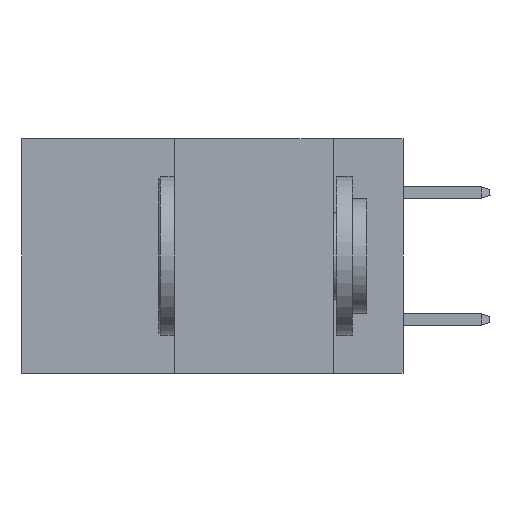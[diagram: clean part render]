
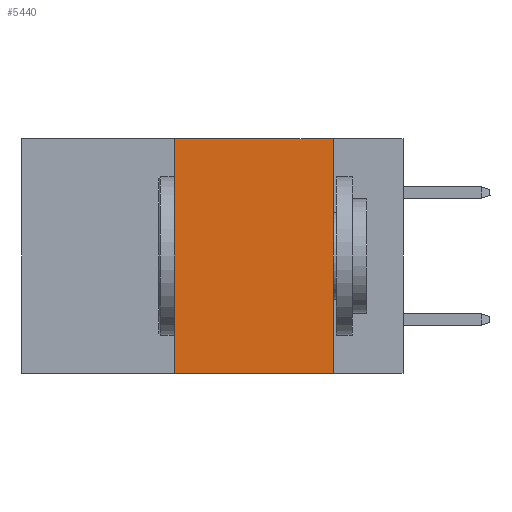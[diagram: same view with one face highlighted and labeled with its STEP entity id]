
A CAD part, left-side view. The second image highlights one B-rep face of the part: STEP entity #5440.
In plain terms, the highlighted planar face has unit normal (-1, 0, 0).
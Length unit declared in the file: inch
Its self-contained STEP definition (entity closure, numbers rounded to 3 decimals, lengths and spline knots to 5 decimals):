
#438 = LINE ( 'NONE', #31145, #23617 ) ;
#1803 = ORIENTED_EDGE ( 'NONE', *, *, #20326, .T. ) ;
#1824 = EDGE_CURVE ( 'NONE', #14585, #17282, #27215, .T. ) ;
#3173 = ORIENTED_EDGE ( 'NONE', *, *, #5258, .F. ) ;
#4298 = VECTOR ( 'NONE', #18772, 39.37008 ) ;
#5089 = LINE ( 'NONE', #29162, #16202 ) ;
#5258 = EDGE_CURVE ( 'NONE', #20251, #14585, #438, .T. ) ;
#5440 = ADVANCED_FACE ( 'NONE', ( #6711 ), #23041, .F. ) ;
#6154 = ORIENTED_EDGE ( 'NONE', *, *, #1824, .F. ) ;
#6711 = FACE_OUTER_BOUND ( 'NONE', #15153, .T. ) ;
#6985 = DIRECTION ( 'NONE',  ( 0., 0., -1. ) ) ;
#8017 = CARTESIAN_POINT ( 'NONE',  ( 0., 0.6, 0. ) ) ;
#9081 = DIRECTION ( 'NONE',  ( 1., 0., 0. ) ) ;
#11461 = AXIS2_PLACEMENT_3D ( 'NONE', #13363, #9081, #27787 ) ;
#12314 = CARTESIAN_POINT ( 'NONE',  ( 0., 0.11, -0.37 ) ) ;
#13363 = CARTESIAN_POINT ( 'NONE',  ( 0., 0.6, 0. ) ) ;
#13610 = EDGE_CURVE ( 'NONE', #17282, #17150, #5089, .T. ) ;
#14349 = CARTESIAN_POINT ( 'NONE',  ( 0., 0.36, 0. ) ) ;
#14585 = VERTEX_POINT ( 'NONE', #14349 ) ;
#15153 = EDGE_LOOP ( 'NONE', ( #29986, #6154, #3173, #1803 ) ) ;
#16202 = VECTOR ( 'NONE', #6985, 39.37008 ) ;
#17146 = CARTESIAN_POINT ( 'NONE',  ( 0., 0.11, 0. ) ) ;
#17150 = VERTEX_POINT ( 'NONE', #12314 ) ;
#17282 = VERTEX_POINT ( 'NONE', #17146 ) ;
#18772 = DIRECTION ( 'NONE',  ( 0., -1., 0. ) ) ;
#20251 = VERTEX_POINT ( 'NONE', #23208 ) ;
#20326 = EDGE_CURVE ( 'NONE', #20251, #17150, #23675, .T. ) ;
#22999 = VECTOR ( 'NONE', #29733, 39.37008 ) ;
#23041 = PLANE ( 'NONE',  #11461 ) ;
#23208 = CARTESIAN_POINT ( 'NONE',  ( 0., 0.36, -0.37 ) ) ;
#23617 = VECTOR ( 'NONE', #29072, 39.37008 ) ;
#23675 = LINE ( 'NONE', #26079, #4298 ) ;
#26079 = CARTESIAN_POINT ( 'NONE',  ( 0., 0.6, -0.37 ) ) ;
#27215 = LINE ( 'NONE', #8017, #22999 ) ;
#27787 = DIRECTION ( 'NONE',  ( 0., 0., -1. ) ) ;
#29072 = DIRECTION ( 'NONE',  ( 0., 0., 1. ) ) ;
#29162 = CARTESIAN_POINT ( 'NONE',  ( 0., 0.11, 0. ) ) ;
#29733 = DIRECTION ( 'NONE',  ( 0., -1., 0. ) ) ;
#29986 = ORIENTED_EDGE ( 'NONE', *, *, #13610, .F. ) ;
#31145 = CARTESIAN_POINT ( 'NONE',  ( 0., 0.36, 0. ) ) ;
